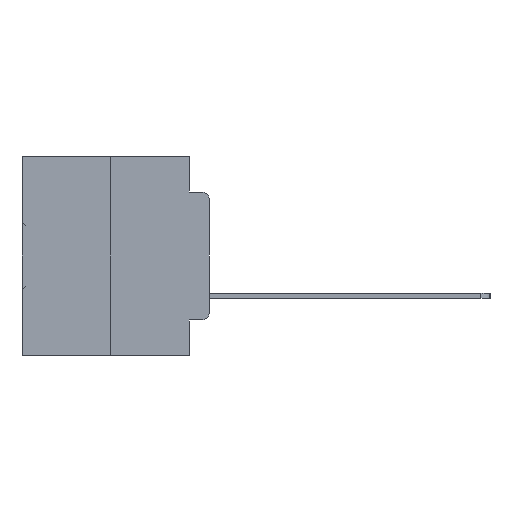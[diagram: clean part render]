
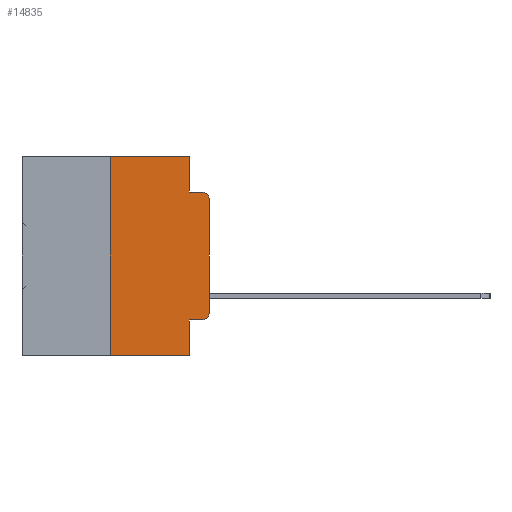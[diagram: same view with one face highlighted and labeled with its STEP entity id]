
A CAD part, left-side view. The second image highlights one B-rep face of the part: STEP entity #14835.
In plain terms, the highlighted planar face has unit normal (-1, 0, 0).
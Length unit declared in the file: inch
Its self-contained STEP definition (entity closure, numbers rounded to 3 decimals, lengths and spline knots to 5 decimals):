
#661 = EDGE_CURVE ( 'NONE', #10179, #22646, #11222, .T. ) ;
#1132 = DIRECTION ( 'NONE',  ( 0., -1., 0. ) ) ;
#1933 = CARTESIAN_POINT ( 'NONE',  ( 0., 0.051, -0.5 ) ) ;
#3308 = VERTEX_POINT ( 'NONE', #12095 ) ;
#4156 = VECTOR ( 'NONE', #5798, 39.37008 ) ;
#4211 = CARTESIAN_POINT ( 'NONE',  ( 0., 0.051, 0. ) ) ;
#4358 = AXIS2_PLACEMENT_3D ( 'NONE', #5481, #24956, #8286 ) ;
#4819 = ORIENTED_EDGE ( 'NONE', *, *, #21383, .T. ) ;
#4947 = ORIENTED_EDGE ( 'NONE', *, *, #10163, .T. ) ;
#4979 = AXIS2_PLACEMENT_3D ( 'NONE', #31426, #28973, #12490 ) ;
#5110 = ORIENTED_EDGE ( 'NONE', *, *, #8265, .F. ) ;
#5272 = EDGE_CURVE ( 'NONE', #28324, #20017, #33038, .T. ) ;
#5481 = CARTESIAN_POINT ( 'NONE',  ( 0., 0.02, -0.1085 ) ) ;
#5569 = ORIENTED_EDGE ( 'NONE', *, *, #661, .F. ) ;
#5798 = DIRECTION ( 'NONE',  ( 0., -1., 0. ) ) ;
#6365 = ORIENTED_EDGE ( 'NONE', *, *, #15744, .F. ) ;
#6545 = CARTESIAN_POINT ( 'NONE',  ( 0., 0.25, 0. ) ) ;
#6590 = ORIENTED_EDGE ( 'NONE', *, *, #34657, .F. ) ;
#6672 = DIRECTION ( 'NONE',  ( 0., 0., 1. ) ) ;
#6953 = ORIENTED_EDGE ( 'NONE', *, *, #5272, .T. ) ;
#7062 = ORIENTED_EDGE ( 'NONE', *, *, #27545, .F. ) ;
#7064 = DIRECTION ( 'NONE',  ( 0., 0., -1. ) ) ;
#7175 = ORIENTED_EDGE ( 'NONE', *, *, #25726, .T. ) ;
#7455 = LINE ( 'NONE', #6545, #28675 ) ;
#7501 = CARTESIAN_POINT ( 'NONE',  ( 0., 0.25, -0.5 ) ) ;
#7520 = ORIENTED_EDGE ( 'NONE', *, *, #14659, .T. ) ;
#8265 = EDGE_CURVE ( 'NONE', #22646, #24319, #13587, .T. ) ;
#8286 = DIRECTION ( 'NONE',  ( 0., 0., -1. ) ) ;
#8932 = CARTESIAN_POINT ( 'NONE',  ( 0., 0.02, -0.3915 ) ) ;
#9652 = PLANE ( 'NONE',  #4979 ) ;
#10093 = DIRECTION ( 'NONE',  ( 0., -1., 0. ) ) ;
#10163 = EDGE_CURVE ( 'NONE', #3308, #24319, #27664, .T. ) ;
#10179 = VERTEX_POINT ( 'NONE', #22324 ) ;
#10695 = VERTEX_POINT ( 'NONE', #32760 ) ;
#11222 = LINE ( 'NONE', #29868, #32227 ) ;
#11771 = DIRECTION ( 'NONE',  ( 0., 0., -1. ) ) ;
#12091 = VECTOR ( 'NONE', #10093, 39.37008 ) ;
#12095 = CARTESIAN_POINT ( 'NONE',  ( 0., 0., -0.1085 ) ) ;
#12490 = DIRECTION ( 'NONE',  ( 0., 0., -1. ) ) ;
#13587 = LINE ( 'NONE', #34228, #20985 ) ;
#13803 = CARTESIAN_POINT ( 'NONE',  ( 0., 0.25, 0. ) ) ;
#14133 = CARTESIAN_POINT ( 'NONE',  ( 0., 0.051, -0.4115 ) ) ;
#14659 = EDGE_CURVE ( 'NONE', #35373, #30849, #31928, .T. ) ;
#14835 = ADVANCED_FACE ( 'NONE', ( #28595 ), #9652, .F. ) ;
#15013 = CARTESIAN_POINT ( 'NONE',  ( 0., 0., 0. ) ) ;
#15209 = VECTOR ( 'NONE', #22031, 39.37008 ) ;
#15744 = EDGE_CURVE ( 'NONE', #34508, #10179, #22590, .T. ) ;
#16451 = CARTESIAN_POINT ( 'NONE',  ( 0., 0.473, 0. ) ) ;
#16959 = AXIS2_PLACEMENT_3D ( 'NONE', #8932, #28286, #11771 ) ;
#17017 = VECTOR ( 'NONE', #31388, 39.37008 ) ;
#17632 = VECTOR ( 'NONE', #7064, 39.37008 ) ;
#17887 = EDGE_LOOP ( 'NONE', ( #4819, #4947, #5110, #5569, #6365, #6590, #6953, #7062, #7175, #7520 ) ) ;
#20017 = VERTEX_POINT ( 'NONE', #1933 ) ;
#20985 = VECTOR ( 'NONE', #1132, 39.37008 ) ;
#21383 = EDGE_CURVE ( 'NONE', #30849, #3308, #25189, .T. ) ;
#21586 = CARTESIAN_POINT ( 'NONE',  ( 0., 0., -0.3915 ) ) ;
#22031 = DIRECTION ( 'NONE',  ( 0., -1., 0. ) ) ;
#22324 = CARTESIAN_POINT ( 'NONE',  ( 0., 0.051, 0. ) ) ;
#22590 = LINE ( 'NONE', #16451, #15209 ) ;
#22646 = VERTEX_POINT ( 'NONE', #29223 ) ;
#23831 = CARTESIAN_POINT ( 'NONE',  ( 0., 0.473, -0.5 ) ) ;
#24319 = VERTEX_POINT ( 'NONE', #32496 ) ;
#24956 = DIRECTION ( 'NONE',  ( -1., 0., 0. ) ) ;
#25189 = LINE ( 'NONE', #15013, #17017 ) ;
#25726 = EDGE_CURVE ( 'NONE', #10695, #35373, #33475, .T. ) ;
#26748 = CARTESIAN_POINT ( 'NONE',  ( 0., 0.02, -0.4115 ) ) ;
#27545 = EDGE_CURVE ( 'NONE', #10695, #20017, #32083, .T. ) ;
#27664 = CIRCLE ( 'NONE', #4358, 0.02 ) ;
#28286 = DIRECTION ( 'NONE',  ( -1., 0., 0. ) ) ;
#28324 = VERTEX_POINT ( 'NONE', #7501 ) ;
#28595 = FACE_OUTER_BOUND ( 'NONE', #17887, .T. ) ;
#28675 = VECTOR ( 'NONE', #6672, 39.37008 ) ;
#28973 = DIRECTION ( 'NONE',  ( 1., 0., 0. ) ) ;
#29223 = CARTESIAN_POINT ( 'NONE',  ( 0., 0.051, -0.0885 ) ) ;
#29868 = CARTESIAN_POINT ( 'NONE',  ( 0., 0.051, 0. ) ) ;
#30849 = VERTEX_POINT ( 'NONE', #21586 ) ;
#31388 = DIRECTION ( 'NONE',  ( 0., 0., 1. ) ) ;
#31426 = CARTESIAN_POINT ( 'NONE',  ( 0., 0.473, 0. ) ) ;
#31928 = CIRCLE ( 'NONE', #16959, 0.02 ) ;
#32083 = LINE ( 'NONE', #4211, #17632 ) ;
#32164 = DIRECTION ( 'NONE',  ( 0., 0., -1. ) ) ;
#32227 = VECTOR ( 'NONE', #32164, 39.37008 ) ;
#32496 = CARTESIAN_POINT ( 'NONE',  ( 0., 0.02, -0.0885 ) ) ;
#32760 = CARTESIAN_POINT ( 'NONE',  ( 0., 0.051, -0.4115 ) ) ;
#33038 = LINE ( 'NONE', #23831, #12091 ) ;
#33475 = LINE ( 'NONE', #14133, #4156 ) ;
#34228 = CARTESIAN_POINT ( 'NONE',  ( 0., 0.051, -0.0885 ) ) ;
#34508 = VERTEX_POINT ( 'NONE', #13803 ) ;
#34657 = EDGE_CURVE ( 'NONE', #28324, #34508, #7455, .T. ) ;
#35373 = VERTEX_POINT ( 'NONE', #26748 ) ;
